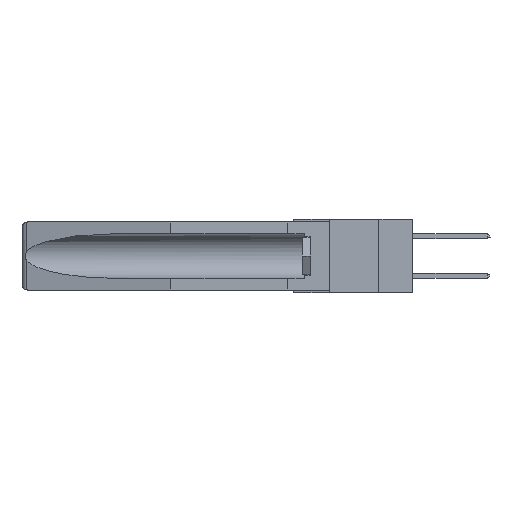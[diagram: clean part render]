
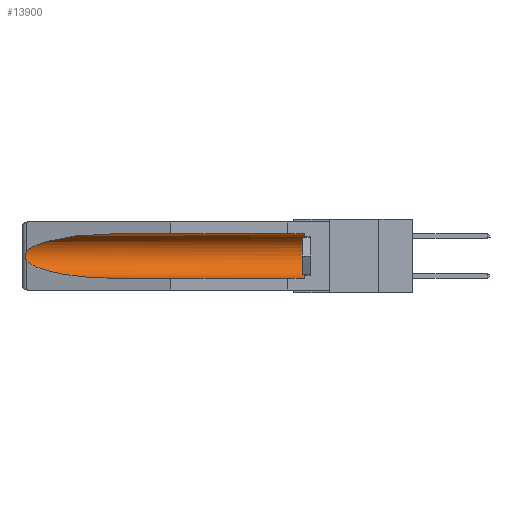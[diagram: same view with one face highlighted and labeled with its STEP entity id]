
A CAD part, left-side view. The second image highlights one B-rep face of the part: STEP entity #13900.
In plain terms, the highlighted cylindrical face has radius 2.857 mm (diameter 5.715 mm), a partial arc.
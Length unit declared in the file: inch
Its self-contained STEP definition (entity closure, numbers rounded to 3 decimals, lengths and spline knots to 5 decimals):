
#43 = CARTESIAN_POINT ( 'NONE',  ( 0.26654, 1.53092, -0.15636 ) ) ;
#488 = CARTESIAN_POINT ( 'NONE',  ( 0.2673, 1.5327, -0.16383 ) ) ;
#1442 = CIRCLE ( 'NONE', #18193, 0.1125 ) ;
#2211 = VERTEX_POINT ( 'NONE', #4615 ) ;
#2226 = CARTESIAN_POINT ( 'NONE',  ( 0.26537, 1.52718, -0.19328 ) ) ;
#2299 = CARTESIAN_POINT ( 'NONE',  ( 0.26655, 1.53094, -0.18657 ) ) ;
#3230 = CARTESIAN_POINT ( 'NONE',  ( 0.25451, 1.48313, -0.09465 ) ) ;
#3349 = EDGE_CURVE ( 'NONE', #22090, #2211, #4936, .T. ) ;
#4453 = VECTOR ( 'NONE', #21936, 39.37008 ) ;
#4608 = EDGE_CURVE ( 'NONE', #7621, #7280, #1442, .T. ) ;
#4615 = CARTESIAN_POINT ( 'NONE',  ( 0.26537, 1.52718, -0.14972 ) ) ;
#4936 =( BOUNDED_CURVE ( )  B_SPLINE_CURVE ( 3, ( #8215, #20355, #3230, #15241 ),
 .UNSPECIFIED., .F., .F. ) 
 B_SPLINE_CURVE_WITH_KNOTS ( ( 4, 4 ),
 ( 4.71239, 6.08839 ),
 .UNSPECIFIED. ) 
 CURVE ( )  GEOMETRIC_REPRESENTATION_ITEM ( )  RATIONAL_B_SPLINE_CURVE ( ( 1., 0.848, 0.848, 1. ) ) 
 REPRESENTATION_ITEM ( '' )  );
#5254 = VERTEX_POINT ( 'NONE', #6808 ) ;
#5335 = FACE_OUTER_BOUND ( 'NONE', #14236, .T. ) ;
#5404 = ORIENTED_EDGE ( 'NONE', *, *, #3349, .T. ) ;
#5881 = CARTESIAN_POINT ( 'NONE',  ( 0.155, 1.07973, -0.284 ) ) ;
#5904 = ORIENTED_EDGE ( 'NONE', *, *, #7439, .T. ) ;
#6662 = ORIENTED_EDGE ( 'NONE', *, *, #11773, .F. ) ;
#6808 = CARTESIAN_POINT ( 'NONE',  ( 0.26537, 1.52718, -0.19328 ) ) ;
#7247 = CARTESIAN_POINT ( 'NONE',  ( 0.155, -0.30754, -0.1715 ) ) ;
#7280 = VERTEX_POINT ( 'NONE', #9082 ) ;
#7439 = EDGE_CURVE ( 'NONE', #7280, #22090, #9005, .T. ) ;
#7621 = VERTEX_POINT ( 'NONE', #20483 ) ;
#7927 =( BOUNDED_CURVE ( )  B_SPLINE_CURVE ( 3, ( #12357, #13881, #15617, #5881 ),
 .UNSPECIFIED., .F., .F. ) 
 B_SPLINE_CURVE_WITH_KNOTS ( ( 4, 4 ),
 ( 0.1948, 1.5708 ),
 .UNSPECIFIED. ) 
 CURVE ( )  GEOMETRIC_REPRESENTATION_ITEM ( )  RATIONAL_B_SPLINE_CURVE ( ( 1., 0.848, 0.848, 1. ) ) 
 REPRESENTATION_ITEM ( '' )  );
#8215 = CARTESIAN_POINT ( 'NONE',  ( 0.155, 1.07973, -0.059 ) ) ;
#9005 = LINE ( 'NONE', #12913, #4453 ) ;
#9082 = CARTESIAN_POINT ( 'NONE',  ( 0.155, 0.126, -0.059 ) ) ;
#10046 = CARTESIAN_POINT ( 'NONE',  ( 0.155, -0.30754, -0.284 ) ) ;
#10310 = CARTESIAN_POINT ( 'NONE',  ( 0.26537, 1.52718, -0.14972 ) ) ;
#10750 = CARTESIAN_POINT ( 'NONE',  ( 0.26597, 1.52961, -0.15275 ) ) ;
#11773 = EDGE_CURVE ( 'NONE', #7621, #21082, #19572, .T. ) ;
#12357 = CARTESIAN_POINT ( 'NONE',  ( 0.26537, 1.52718, -0.19328 ) ) ;
#12499 = CARTESIAN_POINT ( 'NONE',  ( 0.2675, 1.53308, -0.17534 ) ) ;
#12590 = CYLINDRICAL_SURFACE ( 'NONE', #12902, 0.1125 ) ;
#12902 = AXIS2_PLACEMENT_3D ( 'NONE', #7247, #21060, #19391 ) ;
#12913 = CARTESIAN_POINT ( 'NONE',  ( 0.155, -0.30754, -0.059 ) ) ;
#13881 = CARTESIAN_POINT ( 'NONE',  ( 0.25451, 1.48313, -0.24835 ) ) ;
#13900 = ADVANCED_FACE ( 'NONE', ( #5335 ), #12590, .F. ) ;
#14236 = EDGE_LOOP ( 'NONE', ( #5404, #16812, #16423, #6662, #20065, #5904 ) ) ;
#14407 = CARTESIAN_POINT ( 'NONE',  ( 0.2673, 1.53269, -0.17917 ) ) ;
#14994 = VECTOR ( 'NONE', #16713, 39.37008 ) ;
#15241 = CARTESIAN_POINT ( 'NONE',  ( 0.26537, 1.52718, -0.14972 ) ) ;
#15289 = B_SPLINE_CURVE_WITH_KNOTS ( 'NONE', 3,
 ( #10310, #10750, #43, #488, #19460, #12499, #14407, #2299, #18986, #2226 ),
 .UNSPECIFIED., .F., .F.,
 ( 4, 2, 2, 2, 4 ),
 ( 0., 0.00029, 0.00058, 0.00087, 0.00117 ),
 .UNSPECIFIED. ) ;
#15617 = CARTESIAN_POINT ( 'NONE',  ( 0.21114, 1.30732, -0.284 ) ) ;
#15849 = CARTESIAN_POINT ( 'NONE',  ( 0.155, 0.126, -0.1715 ) ) ;
#16423 = ORIENTED_EDGE ( 'NONE', *, *, #21194, .T. ) ;
#16521 = CARTESIAN_POINT ( 'NONE',  ( 0.155, 1.07973, -0.059 ) ) ;
#16713 = DIRECTION ( 'NONE',  ( 0., 1., 0. ) ) ;
#16812 = ORIENTED_EDGE ( 'NONE', *, *, #17715, .T. ) ;
#16977 = CARTESIAN_POINT ( 'NONE',  ( 0.155, 1.07973, -0.284 ) ) ;
#17715 = EDGE_CURVE ( 'NONE', #2211, #5254, #15289, .T. ) ;
#18193 = AXIS2_PLACEMENT_3D ( 'NONE', #15849, #20825, #20976 ) ;
#18986 = CARTESIAN_POINT ( 'NONE',  ( 0.26597, 1.5296, -0.19026 ) ) ;
#19391 = DIRECTION ( 'NONE',  ( 0., 0., 1. ) ) ;
#19460 = CARTESIAN_POINT ( 'NONE',  ( 0.2675, 1.53308, -0.16763 ) ) ;
#19572 = LINE ( 'NONE', #10046, #14994 ) ;
#20065 = ORIENTED_EDGE ( 'NONE', *, *, #4608, .T. ) ;
#20355 = CARTESIAN_POINT ( 'NONE',  ( 0.21114, 1.30732, -0.059 ) ) ;
#20483 = CARTESIAN_POINT ( 'NONE',  ( 0.155, 0.126, -0.284 ) ) ;
#20825 = DIRECTION ( 'NONE',  ( 0., -1., 0. ) ) ;
#20976 = DIRECTION ( 'NONE',  ( 0., 0., 1. ) ) ;
#21060 = DIRECTION ( 'NONE',  ( 0., 1., 0. ) ) ;
#21082 = VERTEX_POINT ( 'NONE', #16977 ) ;
#21194 = EDGE_CURVE ( 'NONE', #5254, #21082, #7927, .T. ) ;
#21936 = DIRECTION ( 'NONE',  ( 0., 1., 0. ) ) ;
#22090 = VERTEX_POINT ( 'NONE', #16521 ) ;
